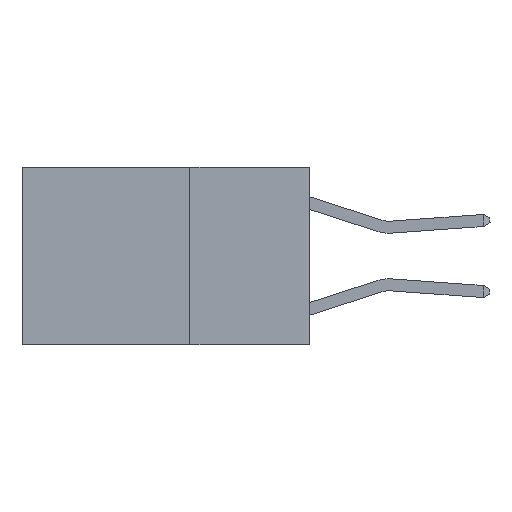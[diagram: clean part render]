
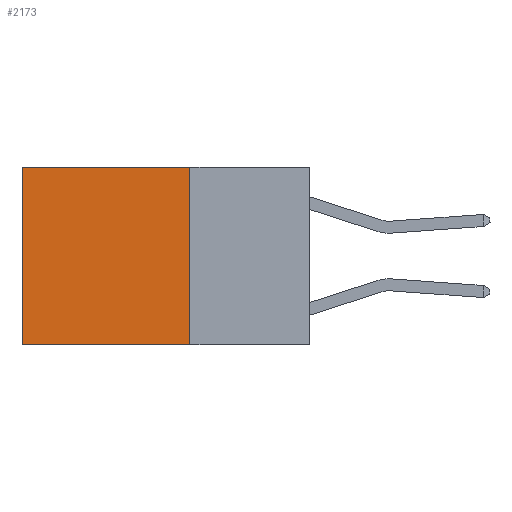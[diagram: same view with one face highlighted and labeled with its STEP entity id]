
A CAD part, left-side view. The second image highlights one B-rep face of the part: STEP entity #2173.
In plain terms, the highlighted planar face has unit normal (-1, 0, 0).
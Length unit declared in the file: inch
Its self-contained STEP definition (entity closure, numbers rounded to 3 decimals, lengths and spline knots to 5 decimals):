
#442 = LINE ( 'NONE', #11334, #11899 ) ;
#1495 = EDGE_CURVE ( 'NONE', #4713, #16516, #442, .T. ) ;
#1988 = LINE ( 'NONE', #4994, #8428 ) ;
#2173 = ADVANCED_FACE ( 'NONE', ( #8481 ), #15696, .F. ) ;
#2821 = EDGE_CURVE ( 'NONE', #4713, #7459, #12534, .T. ) ;
#3256 = EDGE_CURVE ( 'NONE', #16516, #14870, #5234, .T. ) ;
#3551 = DIRECTION ( 'NONE',  ( 0., 0., -1. ) ) ;
#4050 = CARTESIAN_POINT ( 'NONE',  ( 0.2625, 0.25, 0. ) ) ;
#4305 = VECTOR ( 'NONE', #12796, 39.37008 ) ;
#4713 = VERTEX_POINT ( 'NONE', #9843 ) ;
#4765 = VECTOR ( 'NONE', #6529, 39.37008 ) ;
#4994 = CARTESIAN_POINT ( 'NONE',  ( 0.2625, 0.6, 0. ) ) ;
#5234 = LINE ( 'NONE', #6468, #4765 ) ;
#6262 = CARTESIAN_POINT ( 'NONE',  ( 0.2625, 0.6, 0. ) ) ;
#6468 = CARTESIAN_POINT ( 'NONE',  ( 0.2625, 0.25, -0.37 ) ) ;
#6529 = DIRECTION ( 'NONE',  ( 0., 1., 0. ) ) ;
#7137 = CARTESIAN_POINT ( 'NONE',  ( 0.2625, 0.25, 0. ) ) ;
#7459 = VERTEX_POINT ( 'NONE', #6262 ) ;
#8428 = VECTOR ( 'NONE', #3551, 39.37008 ) ;
#8481 = FACE_OUTER_BOUND ( 'NONE', #17539, .T. ) ;
#8595 = DIRECTION ( 'NONE',  ( 0., 0., -1. ) ) ;
#8618 = ORIENTED_EDGE ( 'NONE', *, *, #2821, .T. ) ;
#9729 = AXIS2_PLACEMENT_3D ( 'NONE', #7137, #17095, #8595 ) ;
#9843 = CARTESIAN_POINT ( 'NONE',  ( 0.2625, 0.25, 0. ) ) ;
#9998 = EDGE_CURVE ( 'NONE', #7459, #14870, #1988, .T. ) ;
#11334 = CARTESIAN_POINT ( 'NONE',  ( 0.2625, 0.25, 0. ) ) ;
#11899 = VECTOR ( 'NONE', #14169, 39.37008 ) ;
#12534 = LINE ( 'NONE', #4050, #4305 ) ;
#12796 = DIRECTION ( 'NONE',  ( 0., 1., 0. ) ) ;
#13295 = CARTESIAN_POINT ( 'NONE',  ( 0.2625, 0.25, -0.37 ) ) ;
#14169 = DIRECTION ( 'NONE',  ( 0., 0., -1. ) ) ;
#14562 = CARTESIAN_POINT ( 'NONE',  ( 0.2625, 0.6, -0.37 ) ) ;
#14870 = VERTEX_POINT ( 'NONE', #14562 ) ;
#15696 = PLANE ( 'NONE',  #9729 ) ;
#16516 = VERTEX_POINT ( 'NONE', #13295 ) ;
#17095 = DIRECTION ( 'NONE',  ( 1., 0., 0. ) ) ;
#17539 = EDGE_LOOP ( 'NONE', ( #17748, #18003, #18566, #8618 ) ) ;
#17748 = ORIENTED_EDGE ( 'NONE', *, *, #9998, .T. ) ;
#18003 = ORIENTED_EDGE ( 'NONE', *, *, #3256, .F. ) ;
#18566 = ORIENTED_EDGE ( 'NONE', *, *, #1495, .F. ) ;
